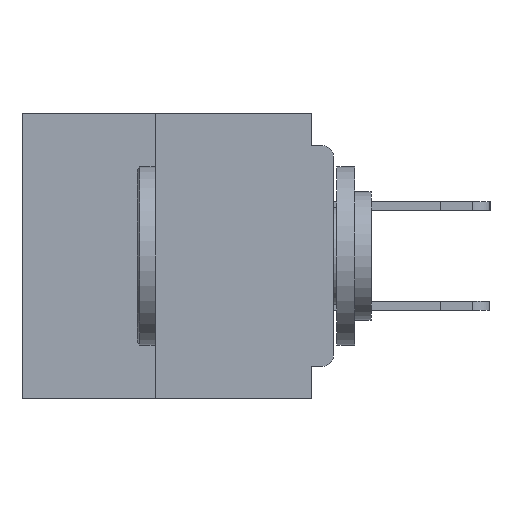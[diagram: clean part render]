
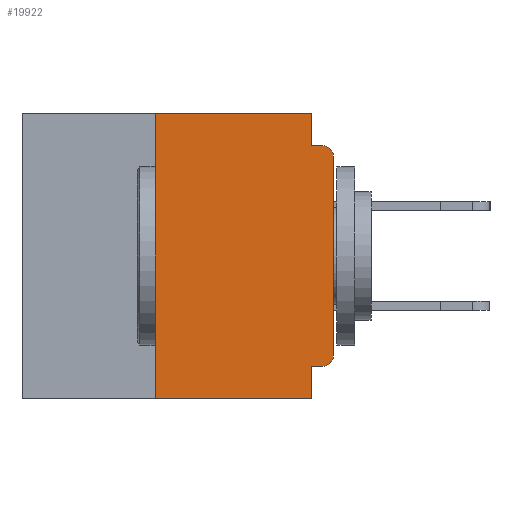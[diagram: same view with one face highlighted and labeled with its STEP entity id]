
A CAD part, left-side view. The second image highlights one B-rep face of the part: STEP entity #19922.
In plain terms, the highlighted planar face has unit normal (-1, 0, 0).
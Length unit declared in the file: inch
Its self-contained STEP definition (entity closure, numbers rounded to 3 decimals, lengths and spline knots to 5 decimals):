
#1278 = EDGE_CURVE ( 'NONE', #19458, #2461, #6624, .T. ) ;
#1943 = DIRECTION ( 'NONE',  ( 0., 0., 1. ) ) ;
#2434 = LINE ( 'NONE', #9290, #47239 ) ;
#2461 = VERTEX_POINT ( 'NONE', #19599 ) ;
#3008 = VERTEX_POINT ( 'NONE', #3508 ) ;
#3033 = CARTESIAN_POINT ( 'NONE',  ( 0., 0.437, 0. ) ) ;
#3423 = PLANE ( 'NONE',  #54860 ) ;
#3508 = CARTESIAN_POINT ( 'NONE',  ( 0., 0.031, 0. ) ) ;
#3516 = AXIS2_PLACEMENT_3D ( 'NONE', #49084, #23184, #53369 ) ;
#3679 = ORIENTED_EDGE ( 'NONE', *, *, #15356, .T. ) ;
#4788 = ORIENTED_EDGE ( 'NONE', *, *, #16063, .F. ) ;
#4899 = DIRECTION ( 'NONE',  ( 0., -1., 0. ) ) ;
#6620 = ORIENTED_EDGE ( 'NONE', *, *, #37257, .F. ) ;
#6624 = CIRCLE ( 'NONE', #55903, 0.015 ) ;
#7823 = DIRECTION ( 'NONE',  ( 0., 0., -1. ) ) ;
#8440 = ORIENTED_EDGE ( 'NONE', *, *, #33314, .T. ) ;
#9013 = CARTESIAN_POINT ( 'NONE',  ( 0., 0.015, -0.355 ) ) ;
#9290 = CARTESIAN_POINT ( 'NONE',  ( 0., 0.437, -0.4 ) ) ;
#10556 = CARTESIAN_POINT ( 'NONE',  ( 0., 0.031, -0.4 ) ) ;
#10717 = LINE ( 'NONE', #3033, #55383 ) ;
#12605 = CARTESIAN_POINT ( 'NONE',  ( 0., 0.031, -0.355 ) ) ;
#13290 = ORIENTED_EDGE ( 'NONE', *, *, #45199, .T. ) ;
#14428 = VECTOR ( 'NONE', #40924, 39.37008 ) ;
#14502 = LINE ( 'NONE', #14924, #24662 ) ;
#14924 = CARTESIAN_POINT ( 'NONE',  ( 0., 0., 0. ) ) ;
#15356 = EDGE_CURVE ( 'NONE', #41853, #54277, #39633, .T. ) ;
#15547 = DIRECTION ( 'NONE',  ( 0., 1., 0. ) ) ;
#16063 = EDGE_CURVE ( 'NONE', #45496, #44277, #24592, .T. ) ;
#19458 = VERTEX_POINT ( 'NONE', #9013 ) ;
#19599 = CARTESIAN_POINT ( 'NONE',  ( 0., 0., -0.34 ) ) ;
#19922 = ADVANCED_FACE ( 'NONE', ( #34774 ), #3423, .F. ) ;
#19997 = ORIENTED_EDGE ( 'NONE', *, *, #48647, .F. ) ;
#21400 = ORIENTED_EDGE ( 'NONE', *, *, #28288, .F. ) ;
#21629 = DIRECTION ( 'NONE',  ( 0., 0., -1. ) ) ;
#21756 = CARTESIAN_POINT ( 'NONE',  ( 0., 0.031, -0.045 ) ) ;
#21886 = CARTESIAN_POINT ( 'NONE',  ( 0., 0.25, -0.4 ) ) ;
#22392 = CARTESIAN_POINT ( 'NONE',  ( 0., 0.015, -0.045 ) ) ;
#23184 = DIRECTION ( 'NONE',  ( -1., 0., 0. ) ) ;
#24032 = VERTEX_POINT ( 'NONE', #24909 ) ;
#24592 = LINE ( 'NONE', #10556, #14428 ) ;
#24662 = VECTOR ( 'NONE', #1943, 39.37008 ) ;
#24909 = CARTESIAN_POINT ( 'NONE',  ( 0., 0.25, 0. ) ) ;
#26851 = VERTEX_POINT ( 'NONE', #47780 ) ;
#26957 = VECTOR ( 'NONE', #54105, 39.37008 ) ;
#27472 = EDGE_CURVE ( 'NONE', #3008, #29562, #50726, .T. ) ;
#27592 = LINE ( 'NONE', #41316, #37763 ) ;
#28044 = EDGE_CURVE ( 'NONE', #24032, #3008, #10717, .T. ) ;
#28185 = CARTESIAN_POINT ( 'NONE',  ( 0., 0., -0.06 ) ) ;
#28288 = EDGE_CURVE ( 'NONE', #26851, #24032, #56047, .T. ) ;
#28320 = LINE ( 'NONE', #36801, #26957 ) ;
#29435 = CARTESIAN_POINT ( 'NONE',  ( 0., 0.437, 0. ) ) ;
#29562 = VERTEX_POINT ( 'NONE', #21756 ) ;
#30514 = VECTOR ( 'NONE', #21629, 39.37008 ) ;
#31866 = CARTESIAN_POINT ( 'NONE',  ( 0., 0.031, -0.4 ) ) ;
#32455 = EDGE_LOOP ( 'NONE', ( #13290, #3679, #19997, #42515, #55612, #21400, #8440, #4788, #6620, #53711 ) ) ;
#33314 = EDGE_CURVE ( 'NONE', #26851, #44277, #2434, .T. ) ;
#33799 = DIRECTION ( 'NONE',  ( 1., 0., 0. ) ) ;
#34774 = FACE_OUTER_BOUND ( 'NONE', #32455, .T. ) ;
#36801 = CARTESIAN_POINT ( 'NONE',  ( 0., 0., -0.045 ) ) ;
#37257 = EDGE_CURVE ( 'NONE', #19458, #45496, #27592, .T. ) ;
#37763 = VECTOR ( 'NONE', #15547, 39.37008 ) ;
#39633 = CIRCLE ( 'NONE', #3516, 0.015 ) ;
#40924 = DIRECTION ( 'NONE',  ( 0., 0., -1. ) ) ;
#41316 = CARTESIAN_POINT ( 'NONE',  ( 0., 0., -0.355 ) ) ;
#41853 = VERTEX_POINT ( 'NONE', #28185 ) ;
#42515 = ORIENTED_EDGE ( 'NONE', *, *, #27472, .F. ) ;
#43617 = DIRECTION ( 'NONE',  ( 0., 0., 1. ) ) ;
#44277 = VERTEX_POINT ( 'NONE', #31866 ) ;
#45199 = EDGE_CURVE ( 'NONE', #2461, #41853, #14502, .T. ) ;
#45496 = VERTEX_POINT ( 'NONE', #12605 ) ;
#46479 = DIRECTION ( 'NONE',  ( 0., -1., 0. ) ) ;
#47239 = VECTOR ( 'NONE', #4899, 39.37008 ) ;
#47780 = CARTESIAN_POINT ( 'NONE',  ( 0., 0.25, -0.4 ) ) ;
#48647 = EDGE_CURVE ( 'NONE', #29562, #54277, #28320, .T. ) ;
#48783 = DIRECTION ( 'NONE',  ( 0., 0., -1. ) ) ;
#48976 = DIRECTION ( 'NONE',  ( -1., 0., 0. ) ) ;
#49084 = CARTESIAN_POINT ( 'NONE',  ( 0., 0.015, -0.06 ) ) ;
#49087 = CARTESIAN_POINT ( 'NONE',  ( 0., 0.015, -0.34 ) ) ;
#50726 = LINE ( 'NONE', #51828, #30514 ) ;
#51828 = CARTESIAN_POINT ( 'NONE',  ( 0., 0.031, 0. ) ) ;
#53369 = DIRECTION ( 'NONE',  ( 0., 0., -1. ) ) ;
#53711 = ORIENTED_EDGE ( 'NONE', *, *, #1278, .T. ) ;
#54105 = DIRECTION ( 'NONE',  ( 0., -1., 0. ) ) ;
#54277 = VERTEX_POINT ( 'NONE', #22392 ) ;
#54677 = VECTOR ( 'NONE', #43617, 39.37008 ) ;
#54860 = AXIS2_PLACEMENT_3D ( 'NONE', #29435, #33799, #7823 ) ;
#55383 = VECTOR ( 'NONE', #46479, 39.37008 ) ;
#55612 = ORIENTED_EDGE ( 'NONE', *, *, #28044, .F. ) ;
#55903 = AXIS2_PLACEMENT_3D ( 'NONE', #49087, #48976, #48783 ) ;
#56047 = LINE ( 'NONE', #21886, #54677 ) ;
